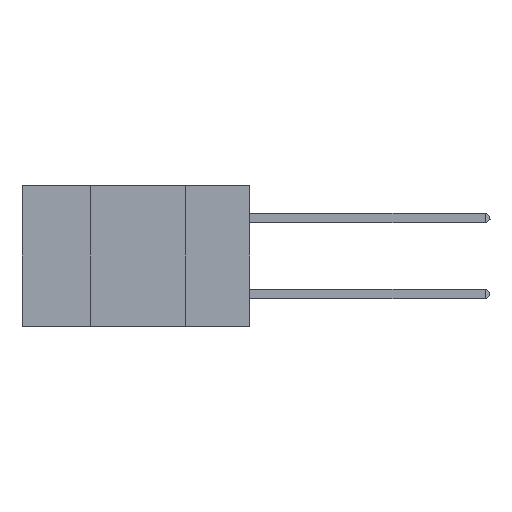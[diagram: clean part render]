
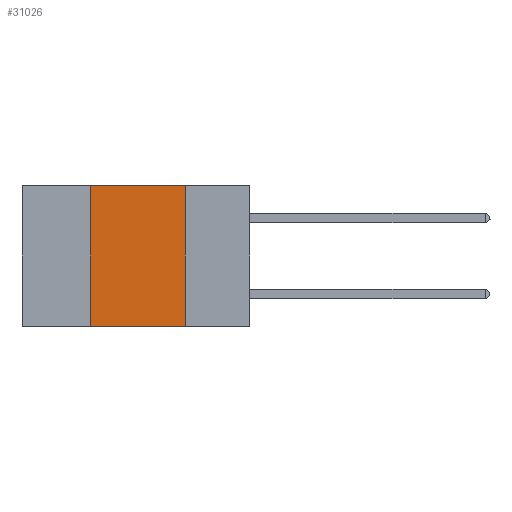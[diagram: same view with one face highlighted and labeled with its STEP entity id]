
A CAD part, left-side view. The second image highlights one B-rep face of the part: STEP entity #31026.
In plain terms, the highlighted planar face has unit normal (-1, 0, 0).
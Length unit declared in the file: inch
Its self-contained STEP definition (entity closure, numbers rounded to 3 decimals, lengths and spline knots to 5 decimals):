
#196 = EDGE_CURVE ( 'NONE', #10789, #3735, #21987, .T. ) ;
#370 = CARTESIAN_POINT ( 'NONE',  ( 0., 0.42, 0. ) ) ;
#1610 = ORIENTED_EDGE ( 'NONE', *, *, #21057, .F. ) ;
#1899 = EDGE_CURVE ( 'NONE', #28709, #3735, #12748, .T. ) ;
#2324 = DIRECTION ( 'NONE',  ( 0., -1., 0. ) ) ;
#2717 = ORIENTED_EDGE ( 'NONE', *, *, #7873, .F. ) ;
#3735 = VERTEX_POINT ( 'NONE', #23973 ) ;
#4195 = VECTOR ( 'NONE', #2324, 39.37008 ) ;
#6623 = DIRECTION ( 'NONE',  ( 0., -1., 0. ) ) ;
#7873 = EDGE_CURVE ( 'NONE', #14346, #10789, #11377, .T. ) ;
#8575 = CARTESIAN_POINT ( 'NONE',  ( 0., 0.17, 0. ) ) ;
#8731 = CARTESIAN_POINT ( 'NONE',  ( 0., 0.6, 0. ) ) ;
#10206 = VECTOR ( 'NONE', #15500, 39.37008 ) ;
#10785 = ORIENTED_EDGE ( 'NONE', *, *, #196, .F. ) ;
#10789 = VERTEX_POINT ( 'NONE', #16060 ) ;
#11377 = LINE ( 'NONE', #8731, #19051 ) ;
#12748 = LINE ( 'NONE', #29305, #4195 ) ;
#13177 = DIRECTION ( 'NONE',  ( 1., 0., 0. ) ) ;
#13179 = CARTESIAN_POINT ( 'NONE',  ( 0., 0.42, 0. ) ) ;
#14346 = VERTEX_POINT ( 'NONE', #370 ) ;
#15500 = DIRECTION ( 'NONE',  ( 0., 0., 1. ) ) ;
#16060 = CARTESIAN_POINT ( 'NONE',  ( 0., 0.17, 0. ) ) ;
#16358 = PLANE ( 'NONE',  #23858 ) ;
#19051 = VECTOR ( 'NONE', #6623, 39.37008 ) ;
#21057 = EDGE_CURVE ( 'NONE', #28709, #14346, #28887, .T. ) ;
#21987 = LINE ( 'NONE', #8575, #22071 ) ;
#22071 = VECTOR ( 'NONE', #24443, 39.37008 ) ;
#23858 = AXIS2_PLACEMENT_3D ( 'NONE', #24463, #13177, #34508 ) ;
#23973 = CARTESIAN_POINT ( 'NONE',  ( 0., 0.17, -0.37 ) ) ;
#24443 = DIRECTION ( 'NONE',  ( 0., 0., -1. ) ) ;
#24463 = CARTESIAN_POINT ( 'NONE',  ( 0., 0.6, 0. ) ) ;
#28709 = VERTEX_POINT ( 'NONE', #31609 ) ;
#28887 = LINE ( 'NONE', #13179, #10206 ) ;
#29305 = CARTESIAN_POINT ( 'NONE',  ( 0., 0.6, -0.37 ) ) ;
#29578 = FACE_OUTER_BOUND ( 'NONE', #31373, .T. ) ;
#31026 = ADVANCED_FACE ( 'NONE', ( #29578 ), #16358, .F. ) ;
#31373 = EDGE_LOOP ( 'NONE', ( #10785, #2717, #1610, #34632 ) ) ;
#31609 = CARTESIAN_POINT ( 'NONE',  ( 0., 0.42, -0.37 ) ) ;
#34508 = DIRECTION ( 'NONE',  ( 0., 0., -1. ) ) ;
#34632 = ORIENTED_EDGE ( 'NONE', *, *, #1899, .T. ) ;
